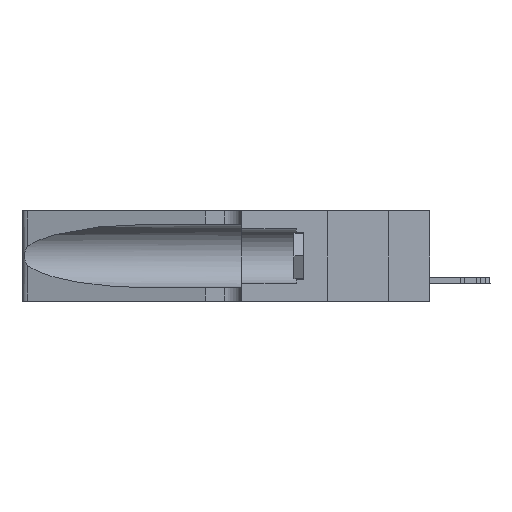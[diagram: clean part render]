
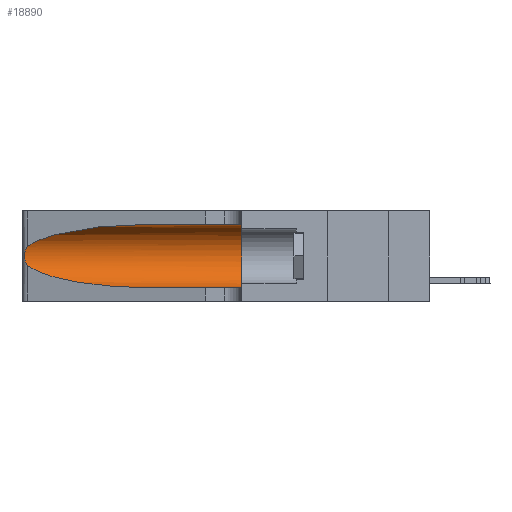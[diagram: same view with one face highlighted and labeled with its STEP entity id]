
A CAD part, left-side view. The second image highlights one B-rep face of the part: STEP entity #18890.
In plain terms, the highlighted cylindrical face has radius 3.308 mm (diameter 6.617 mm), a partial arc.
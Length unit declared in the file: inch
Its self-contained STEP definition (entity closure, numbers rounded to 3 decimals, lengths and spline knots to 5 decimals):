
#376 = CARTESIAN_POINT ( 'NONE',  ( 0.25854, 1.2359, 0.20912 ) ) ;
#524 = CARTESIAN_POINT ( 'NONE',  ( 0.26075, 1.23896, 0.178 ) ) ;
#3588 = EDGE_LOOP ( 'NONE', ( #5182, #39905, #38252, #4844, #21659, #4334 ) ) ;
#3609 = DIRECTION ( 'NONE',  ( 0., 1., 0. ) ) ;
#3814 = CARTESIAN_POINT ( 'NONE',  ( 0.25555, 1.22993, 0.14849 ) ) ;
#4314 = CARTESIAN_POINT ( 'NONE',  ( 0.2373, 1.15595, 0.08982 ) ) ;
#4334 = ORIENTED_EDGE ( 'NONE', *, *, #16272, .F. ) ;
#4844 = ORIENTED_EDGE ( 'NONE', *, *, #6434, .T. ) ;
#5182 = ORIENTED_EDGE ( 'NONE', *, *, #32908, .T. ) ;
#5786 = CARTESIAN_POINT ( 'NONE',  ( 0.25487, 1.22718, 0.22369 ) ) ;
#6130 =( BOUNDED_CURVE ( )  B_SPLINE_CURVE ( 3, ( #31168, #4314, #41012, #24229 ),
 .UNSPECIFIED., .F., .T. ) 
 B_SPLINE_CURVE_WITH_KNOTS ( ( 4, 4 ),
 ( 3.44316, 4.71239 ),
 .UNSPECIFIED. ) 
 CURVE ( )  GEOMETRIC_REPRESENTATION_ITEM ( )  RATIONAL_B_SPLINE_CURVE ( ( 1., 0.87, 0.87, 1. ) ) 
 REPRESENTATION_ITEM ( '' )  );
#6366 = CARTESIAN_POINT ( 'NONE',  ( 0.2373, 1.15595, 0.28018 ) ) ;
#6434 = EDGE_CURVE ( 'NONE', #15262, #10666, #29814, .T. ) ;
#7812 = DIRECTION ( 'NONE',  ( 0., 0., 1. ) ) ;
#8818 = EDGE_CURVE ( 'NONE', #13550, #13156, #32364, .T. ) ;
#10666 = VERTEX_POINT ( 'NONE', #17760 ) ;
#11719 = EDGE_CURVE ( 'NONE', #30106, #10666, #33625, .T. ) ;
#12157 = DIRECTION ( 'NONE',  ( 0., -1., 0. ) ) ;
#12322 = CARTESIAN_POINT ( 'NONE',  ( 0.1305, 1.61858, 0.31525 ) ) ;
#13120 = CARTESIAN_POINT ( 'NONE',  ( 0.25487, 1.22718, 0.14631 ) ) ;
#13156 = VERTEX_POINT ( 'NONE', #13120 ) ;
#13550 = VERTEX_POINT ( 'NONE', #19262 ) ;
#13794 = CARTESIAN_POINT ( 'NONE',  ( 0.1305, 0.72297, 0.31525 ) ) ;
#14428 = CARTESIAN_POINT ( 'NONE',  ( 0.25856, 1.23593, 0.16098 ) ) ;
#15048 = VECTOR ( 'NONE', #25919, 39.37008 ) ;
#15262 = VERTEX_POINT ( 'NONE', #20983 ) ;
#15981 = CARTESIAN_POINT ( 'NONE',  ( 0.25487, 1.22718, 0.22369 ) ) ;
#16050 = DIRECTION ( 'NONE',  ( 0., 0., -1. ) ) ;
#16272 = EDGE_CURVE ( 'NONE', #34292, #30106, #43537, .T. ) ;
#16325 = CARTESIAN_POINT ( 'NONE',  ( 0.1305, 0.72297, 0.31525 ) ) ;
#16469 = CARTESIAN_POINT ( 'NONE',  ( 0.18966, 0.96281, 0.31525 ) ) ;
#17123 = CARTESIAN_POINT ( 'NONE',  ( 0.25639, 1.23186, 0.15144 ) ) ;
#17663 = CARTESIAN_POINT ( 'NONE',  ( 0.25789, 1.23486, 0.15765 ) ) ;
#17760 = CARTESIAN_POINT ( 'NONE',  ( 0.1305, 0.35, 0.05475 ) ) ;
#18507 = CYLINDRICAL_SURFACE ( 'NONE', #35034, 0.13025 ) ;
#18890 = ADVANCED_FACE ( 'NONE', ( #21633 ), #18507, .F. ) ;
#19262 = CARTESIAN_POINT ( 'NONE',  ( 0.25487, 1.22718, 0.22369 ) ) ;
#19952 = CARTESIAN_POINT ( 'NONE',  ( 0.1305, 0.35, 0.31525 ) ) ;
#20016 = CARTESIAN_POINT ( 'NONE',  ( 0.1305, 0.35, 0.185 ) ) ;
#20631 = CARTESIAN_POINT ( 'NONE',  ( 0.25787, 1.23484, 0.2124 ) ) ;
#20983 = CARTESIAN_POINT ( 'NONE',  ( 0.1305, 0.72297, 0.05475 ) ) ;
#21259 =( BOUNDED_CURVE ( )  B_SPLINE_CURVE ( 3, ( #16325, #16469, #6366, #5786 ),
 .UNSPECIFIED., .F., .T. ) 
 B_SPLINE_CURVE_WITH_KNOTS ( ( 4, 4 ),
 ( 1.5708, 2.84003 ),
 .UNSPECIFIED. ) 
 CURVE ( )  GEOMETRIC_REPRESENTATION_ITEM ( )  RATIONAL_B_SPLINE_CURVE ( ( 1., 0.87, 0.87, 1. ) ) 
 REPRESENTATION_ITEM ( '' )  );
#21633 = FACE_OUTER_BOUND ( 'NONE', #3588, .T. ) ;
#21659 = ORIENTED_EDGE ( 'NONE', *, *, #11719, .F. ) ;
#21854 = VECTOR ( 'NONE', #29494, 39.37008 ) ;
#24018 = CARTESIAN_POINT ( 'NONE',  ( 0.26017, 1.23833, 0.17102 ) ) ;
#24229 = CARTESIAN_POINT ( 'NONE',  ( 0.1305, 0.72297, 0.05475 ) ) ;
#25298 = CARTESIAN_POINT ( 'NONE',  ( 0.1305, 1.61858, 0.185 ) ) ;
#25919 = DIRECTION ( 'NONE',  ( 0., -1., 0. ) ) ;
#27561 = CARTESIAN_POINT ( 'NONE',  ( 0.26075, 1.23896, 0.19203 ) ) ;
#29494 = DIRECTION ( 'NONE',  ( 0., -1., 0. ) ) ;
#29814 = LINE ( 'NONE', #35060, #21854 ) ;
#30106 = VERTEX_POINT ( 'NONE', #19952 ) ;
#31168 = CARTESIAN_POINT ( 'NONE',  ( 0.25487, 1.22718, 0.14631 ) ) ;
#32364 = B_SPLINE_CURVE_WITH_KNOTS ( 'NONE', 3,
 ( #15981, #39534, #34611, #20631, #376, #40934, #27561, #524, #24018, #14428, #17663, #17123, #3814, #40659 ),
 .UNSPECIFIED., .F., .F.,
 ( 4, 2, 2, 2, 2, 2, 4 ),
 ( 0., 0.00027, 0.00053, 0.00107, 0.0016, 0.00187, 0.00214 ),
 .UNSPECIFIED. ) ;
#32602 = AXIS2_PLACEMENT_3D ( 'NONE', #20016, #3609, #7812 ) ;
#32908 = EDGE_CURVE ( 'NONE', #34292, #13550, #21259, .T. ) ;
#33625 = CIRCLE ( 'NONE', #32602, 0.13025 ) ;
#34292 = VERTEX_POINT ( 'NONE', #13794 ) ;
#34611 = CARTESIAN_POINT ( 'NONE',  ( 0.25639, 1.23184, 0.21858 ) ) ;
#35034 = AXIS2_PLACEMENT_3D ( 'NONE', #25298, #12157, #16050 ) ;
#35060 = CARTESIAN_POINT ( 'NONE',  ( 0.1305, 1.61858, 0.05475 ) ) ;
#36958 = EDGE_CURVE ( 'NONE', #13156, #15262, #6130, .T. ) ;
#38252 = ORIENTED_EDGE ( 'NONE', *, *, #36958, .T. ) ;
#39534 = CARTESIAN_POINT ( 'NONE',  ( 0.25555, 1.22994, 0.2215 ) ) ;
#39905 = ORIENTED_EDGE ( 'NONE', *, *, #8818, .T. ) ;
#40659 = CARTESIAN_POINT ( 'NONE',  ( 0.25487, 1.22718, 0.14631 ) ) ;
#40934 = CARTESIAN_POINT ( 'NONE',  ( 0.26018, 1.23835, 0.19895 ) ) ;
#41012 = CARTESIAN_POINT ( 'NONE',  ( 0.18966, 0.96281, 0.05475 ) ) ;
#43537 = LINE ( 'NONE', #12322, #15048 ) ;
